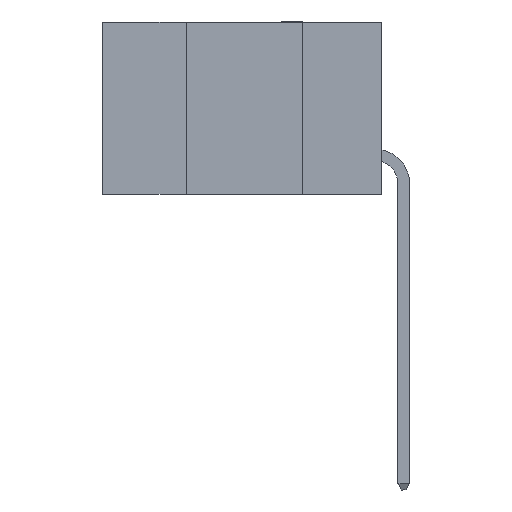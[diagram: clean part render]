
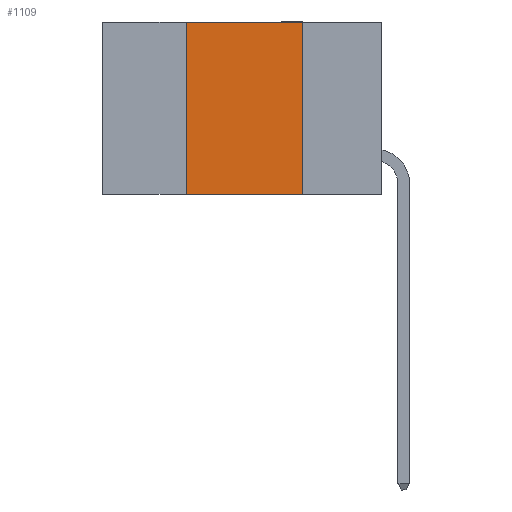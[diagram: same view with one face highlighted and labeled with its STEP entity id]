
A CAD part, left-side view. The second image highlights one B-rep face of the part: STEP entity #1109.
In plain terms, the highlighted planar face has unit normal (-1, 0, 0).
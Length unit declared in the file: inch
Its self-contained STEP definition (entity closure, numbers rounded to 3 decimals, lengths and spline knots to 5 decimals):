
#340 = CARTESIAN_POINT ( 'NONE',  ( 0., 0.42, 0. ) ) ;
#1109 = ADVANCED_FACE ( 'NONE', ( #3835 ), #16001, .F. ) ;
#1641 = VECTOR ( 'NONE', #8667, 39.37008 ) ;
#3279 = VERTEX_POINT ( 'NONE', #4223 ) ;
#3835 = FACE_OUTER_BOUND ( 'NONE', #10807, .T. ) ;
#4223 = CARTESIAN_POINT ( 'NONE',  ( 0., 0.42, -0.37 ) ) ;
#6109 = ORIENTED_EDGE ( 'NONE', *, *, #6932, .F. ) ;
#6178 = CARTESIAN_POINT ( 'NONE',  ( 0., 0.6, 0. ) ) ;
#6573 = DIRECTION ( 'NONE',  ( 1., 0., 0. ) ) ;
#6932 = EDGE_CURVE ( 'NONE', #3279, #16668, #15616, .T. ) ;
#6970 = CARTESIAN_POINT ( 'NONE',  ( 0., 0.6, 0. ) ) ;
#8667 = DIRECTION ( 'NONE',  ( 0., 0., -1. ) ) ;
#9017 = VECTOR ( 'NONE', #13875, 39.37008 ) ;
#9057 = EDGE_CURVE ( 'NONE', #3279, #12902, #9422, .T. ) ;
#9205 = ORIENTED_EDGE ( 'NONE', *, *, #13808, .F. ) ;
#9422 = LINE ( 'NONE', #9929, #9017 ) ;
#9929 = CARTESIAN_POINT ( 'NONE',  ( 0., 0.6, -0.37 ) ) ;
#10383 = VERTEX_POINT ( 'NONE', #16706 ) ;
#10807 = EDGE_LOOP ( 'NONE', ( #14940, #9205, #6109, #14337 ) ) ;
#12060 = LINE ( 'NONE', #6970, #12464 ) ;
#12194 = VECTOR ( 'NONE', #14919, 39.37008 ) ;
#12407 = DIRECTION ( 'NONE',  ( 0., 0., -1. ) ) ;
#12464 = VECTOR ( 'NONE', #16122, 39.37008 ) ;
#12902 = VERTEX_POINT ( 'NONE', #15556 ) ;
#13604 = CARTESIAN_POINT ( 'NONE',  ( 0., 0.42, 0. ) ) ;
#13710 = AXIS2_PLACEMENT_3D ( 'NONE', #6178, #6573, #12407 ) ;
#13808 = EDGE_CURVE ( 'NONE', #16668, #10383, #12060, .T. ) ;
#13875 = DIRECTION ( 'NONE',  ( 0., -1., 0. ) ) ;
#14337 = ORIENTED_EDGE ( 'NONE', *, *, #9057, .T. ) ;
#14919 = DIRECTION ( 'NONE',  ( 0., 0., 1. ) ) ;
#14940 = ORIENTED_EDGE ( 'NONE', *, *, #15710, .F. ) ;
#15556 = CARTESIAN_POINT ( 'NONE',  ( 0., 0.17, -0.37 ) ) ;
#15616 = LINE ( 'NONE', #13604, #12194 ) ;
#15710 = EDGE_CURVE ( 'NONE', #10383, #12902, #16007, .T. ) ;
#16001 = PLANE ( 'NONE',  #13710 ) ;
#16007 = LINE ( 'NONE', #16459, #1641 ) ;
#16122 = DIRECTION ( 'NONE',  ( 0., -1., 0. ) ) ;
#16459 = CARTESIAN_POINT ( 'NONE',  ( 0., 0.17, 0. ) ) ;
#16668 = VERTEX_POINT ( 'NONE', #340 ) ;
#16706 = CARTESIAN_POINT ( 'NONE',  ( 0., 0.17, 0. ) ) ;
